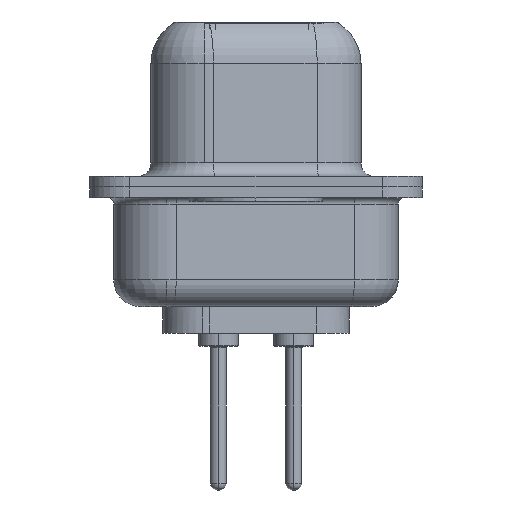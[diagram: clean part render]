
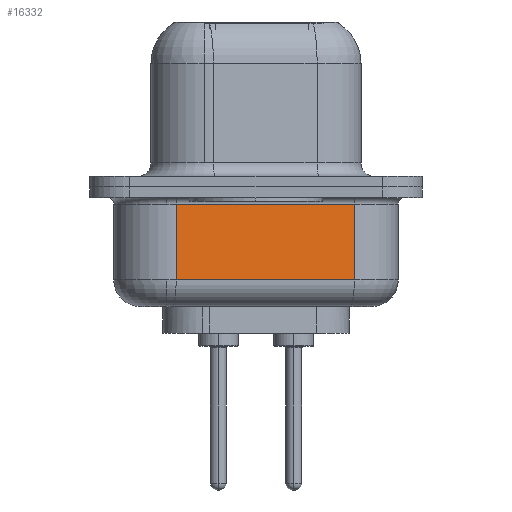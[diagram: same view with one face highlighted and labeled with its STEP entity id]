
A CAD part, left-side view. The second image highlights one B-rep face of the part: STEP entity #16332.
In plain terms, the highlighted planar face has unit normal (-0.985, -0.174, 0).
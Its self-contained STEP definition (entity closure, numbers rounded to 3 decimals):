
#353 = VECTOR ( 'NONE', #2719, 1000. ) ;
#390 = PLANE ( 'NONE',  #4345 ) ;
#730 = CARTESIAN_POINT ( 'NONE',  ( 2.88, 3.003, -0.65 ) ) ;
#859 = CARTESIAN_POINT ( 'NONE',  ( 2.88, 3.003, -4.5 ) ) ;
#2719 = DIRECTION ( 'NONE',  ( 0., 0., 1. ) ) ;
#4260 = LINE ( 'NONE', #17570, #9797 ) ;
#4334 = LINE ( 'NONE', #859, #353 ) ;
#4345 = AXIS2_PLACEMENT_3D ( 'NONE', #9996, #21418, #19783 ) ;
#5188 = DIRECTION ( 'NONE',  ( 0., 0., 1. ) ) ;
#5444 = VECTOR ( 'NONE', #12379, 1000. ) ;
#5802 = VERTEX_POINT ( 'NONE', #8571 ) ;
#6203 = ORIENTED_EDGE ( 'NONE', *, *, #6385, .T. ) ;
#6385 = EDGE_CURVE ( 'NONE', #15753, #5802, #4260, .T. ) ;
#6514 = ORIENTED_EDGE ( 'NONE', *, *, #8700, .F. ) ;
#7060 = EDGE_LOOP ( 'NONE', ( #6514, #6203, #23203, #11512 ) ) ;
#7353 = VERTEX_POINT ( 'NONE', #730 ) ;
#7792 = EDGE_CURVE ( 'NONE', #19440, #7353, #14267, .T. ) ;
#8328 = VECTOR ( 'NONE', #5188, 1000. ) ;
#8571 = CARTESIAN_POINT ( 'NONE',  ( 4.062, -3.697, -3.5 ) ) ;
#8700 = EDGE_CURVE ( 'NONE', #15753, #7353, #4334, .T. ) ;
#9797 = VECTOR ( 'NONE', #23080, 1000. ) ;
#9996 = CARTESIAN_POINT ( 'NONE',  ( 2.88, 3.003, -4.5 ) ) ;
#11180 = LINE ( 'NONE', #20380, #8328 ) ;
#11512 = ORIENTED_EDGE ( 'NONE', *, *, #7792, .T. ) ;
#12089 = FACE_OUTER_BOUND ( 'NONE', #7060, .T. ) ;
#12379 = DIRECTION ( 'NONE',  ( -0.174, 0.985, 0. ) ) ;
#14267 = LINE ( 'NONE', #21948, #5444 ) ;
#15753 = VERTEX_POINT ( 'NONE', #24579 ) ;
#16332 = ADVANCED_FACE ( 'NONE', ( #12089 ), #390, .F. ) ;
#17051 = EDGE_CURVE ( 'NONE', #5802, #19440, #11180, .T. ) ;
#17570 = CARTESIAN_POINT ( 'NONE',  ( 2.88, 3.003, -3.5 ) ) ;
#19440 = VERTEX_POINT ( 'NONE', #19767 ) ;
#19767 = CARTESIAN_POINT ( 'NONE',  ( 4.062, -3.697, -0.65 ) ) ;
#19783 = DIRECTION ( 'NONE',  ( -0.174, 0.985, 0. ) ) ;
#20380 = CARTESIAN_POINT ( 'NONE',  ( 4.062, -3.697, -4.5 ) ) ;
#21418 = DIRECTION ( 'NONE',  ( 0.985, 0.174, 0. ) ) ;
#21948 = CARTESIAN_POINT ( 'NONE',  ( 2.88, 3.003, -0.65 ) ) ;
#23080 = DIRECTION ( 'NONE',  ( 0.174, -0.985, 0. ) ) ;
#23203 = ORIENTED_EDGE ( 'NONE', *, *, #17051, .T. ) ;
#24579 = CARTESIAN_POINT ( 'NONE',  ( 2.88, 3.003, -3.5 ) ) ;
